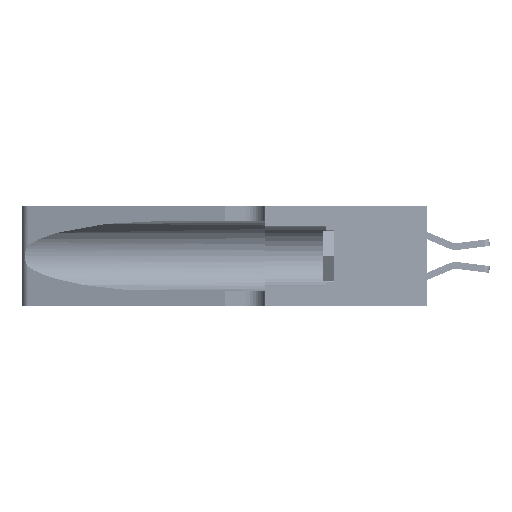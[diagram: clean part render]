
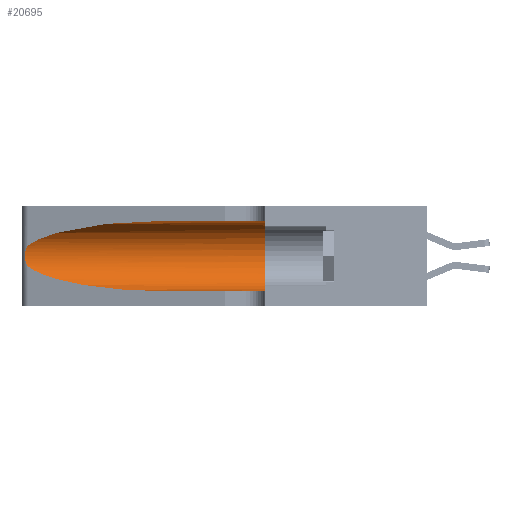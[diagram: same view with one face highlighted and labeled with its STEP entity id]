
A CAD part, left-side view. The second image highlights one B-rep face of the part: STEP entity #20695.
In plain terms, the highlighted cylindrical face has radius 3.308 mm (diameter 6.617 mm), a partial arc.
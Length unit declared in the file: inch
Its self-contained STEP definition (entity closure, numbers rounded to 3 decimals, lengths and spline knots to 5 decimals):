
#72 =( BOUNDED_CURVE ( )  B_SPLINE_CURVE ( 3, ( #38834, #30930, #3303, #15257 ),
 .UNSPECIFIED., .F., .T. ) 
 B_SPLINE_CURVE_WITH_KNOTS ( ( 4, 4 ),
 ( 3.44316, 4.71239 ),
 .UNSPECIFIED. ) 
 CURVE ( )  GEOMETRIC_REPRESENTATION_ITEM ( )  RATIONAL_B_SPLINE_CURVE ( ( 1., 0.87, 0.87, 1. ) ) 
 REPRESENTATION_ITEM ( '' )  );
#582 = CARTESIAN_POINT ( 'NONE',  ( 0.25487, 1.22718, 0.22369 ) ) ;
#637 = VERTEX_POINT ( 'NONE', #31780 ) ;
#1636 = VERTEX_POINT ( 'NONE', #5825 ) ;
#1712 = B_SPLINE_CURVE_WITH_KNOTS ( 'NONE', 3,
 ( #29789, #17929, #37690, #14088, #41618, #18099, #45593, #22097, #49508, #26073, #2306, #29949, #6310, #33889 ),
 .UNSPECIFIED., .F., .F.,
 ( 4, 2, 2, 2, 2, 2, 4 ),
 ( 0., 0.00027, 0.00053, 0.00107, 0.0016, 0.00187, 0.00214 ),
 .UNSPECIFIED. ) ;
#1868 = ORIENTED_EDGE ( 'NONE', *, *, #41012, .T. ) ;
#2306 = CARTESIAN_POINT ( 'NONE',  ( 0.25789, 1.23486, 0.15765 ) ) ;
#2549 = CARTESIAN_POINT ( 'NONE',  ( 0.1305, 0.35, 0.185 ) ) ;
#3303 = CARTESIAN_POINT ( 'NONE',  ( 0.18966, 0.96281, 0.05475 ) ) ;
#3572 = CARTESIAN_POINT ( 'NONE',  ( 0.25487, 1.22718, 0.14631 ) ) ;
#4910 = VECTOR ( 'NONE', #15289, 39.37008 ) ;
#4964 = EDGE_CURVE ( 'NONE', #38314, #37856, #72, .T. ) ;
#5825 = CARTESIAN_POINT ( 'NONE',  ( 0.1305, 0.72297, 0.31525 ) ) ;
#6018 = ORIENTED_EDGE ( 'NONE', *, *, #34022, .T. ) ;
#6310 = CARTESIAN_POINT ( 'NONE',  ( 0.25555, 1.22993, 0.14849 ) ) ;
#6532 = EDGE_LOOP ( 'NONE', ( #1868, #13918, #30629, #6018, #17808, #25780 ) ) ;
#6535 = DIRECTION ( 'NONE',  ( 0., 0., 1. ) ) ;
#7098 = CARTESIAN_POINT ( 'NONE',  ( 0.1305, 1.61858, 0.185 ) ) ;
#7361 = AXIS2_PLACEMENT_3D ( 'NONE', #2549, #30192, #6535 ) ;
#10018 = EDGE_CURVE ( 'NONE', #1636, #637, #36381, .T. ) ;
#10527 = FACE_OUTER_BOUND ( 'NONE', #6532, .T. ) ;
#12421 = CARTESIAN_POINT ( 'NONE',  ( 0.1305, 0.72297, 0.31525 ) ) ;
#12972 = CARTESIAN_POINT ( 'NONE',  ( 0.1305, 0.72297, 0.05475 ) ) ;
#13918 = ORIENTED_EDGE ( 'NONE', *, *, #26414, .T. ) ;
#14088 = CARTESIAN_POINT ( 'NONE',  ( 0.25787, 1.23484, 0.2124 ) ) ;
#15257 = CARTESIAN_POINT ( 'NONE',  ( 0.1305, 0.72297, 0.05475 ) ) ;
#15289 = DIRECTION ( 'NONE',  ( 0., -1., 0. ) ) ;
#16343 =( BOUNDED_CURVE ( )  B_SPLINE_CURVE ( 3, ( #12421, #36013, #24368, #582 ),
 .UNSPECIFIED., .F., .T. ) 
 B_SPLINE_CURVE_WITH_KNOTS ( ( 4, 4 ),
 ( 1.5708, 2.84003 ),
 .UNSPECIFIED. ) 
 CURVE ( )  GEOMETRIC_REPRESENTATION_ITEM ( )  RATIONAL_B_SPLINE_CURVE ( ( 1., 0.87, 0.87, 1. ) ) 
 REPRESENTATION_ITEM ( '' )  );
#17808 = ORIENTED_EDGE ( 'NONE', *, *, #38100, .F. ) ;
#17929 = CARTESIAN_POINT ( 'NONE',  ( 0.25555, 1.22994, 0.2215 ) ) ;
#18099 = CARTESIAN_POINT ( 'NONE',  ( 0.26018, 1.23835, 0.19895 ) ) ;
#20695 = ADVANCED_FACE ( 'NONE', ( #10527 ), #38252, .F. ) ;
#22097 = CARTESIAN_POINT ( 'NONE',  ( 0.26075, 1.23896, 0.178 ) ) ;
#23934 = DIRECTION ( 'NONE',  ( 0., -1., 0. ) ) ;
#24368 = CARTESIAN_POINT ( 'NONE',  ( 0.2373, 1.15595, 0.28018 ) ) ;
#25780 = ORIENTED_EDGE ( 'NONE', *, *, #10018, .F. ) ;
#26073 = CARTESIAN_POINT ( 'NONE',  ( 0.25856, 1.23593, 0.16098 ) ) ;
#26414 = EDGE_CURVE ( 'NONE', #46879, #38314, #1712, .T. ) ;
#27236 = LINE ( 'NONE', #35767, #37652 ) ;
#29789 = CARTESIAN_POINT ( 'NONE',  ( 0.25487, 1.22718, 0.22369 ) ) ;
#29949 = CARTESIAN_POINT ( 'NONE',  ( 0.25639, 1.23186, 0.15144 ) ) ;
#30192 = DIRECTION ( 'NONE',  ( 0., 1., 0. ) ) ;
#30629 = ORIENTED_EDGE ( 'NONE', *, *, #4964, .T. ) ;
#30930 = CARTESIAN_POINT ( 'NONE',  ( 0.2373, 1.15595, 0.08982 ) ) ;
#31780 = CARTESIAN_POINT ( 'NONE',  ( 0.1305, 0.35, 0.31525 ) ) ;
#33508 = CARTESIAN_POINT ( 'NONE',  ( 0.25487, 1.22718, 0.22369 ) ) ;
#33889 = CARTESIAN_POINT ( 'NONE',  ( 0.25487, 1.22718, 0.14631 ) ) ;
#34022 = EDGE_CURVE ( 'NONE', #37856, #47213, #27236, .T. ) ;
#34691 = DIRECTION ( 'NONE',  ( 0., -1., 0. ) ) ;
#35767 = CARTESIAN_POINT ( 'NONE',  ( 0.1305, 1.61858, 0.05475 ) ) ;
#36013 = CARTESIAN_POINT ( 'NONE',  ( 0.18966, 0.96281, 0.31525 ) ) ;
#36381 = LINE ( 'NONE', #42801, #4910 ) ;
#37652 = VECTOR ( 'NONE', #23934, 39.37008 ) ;
#37690 = CARTESIAN_POINT ( 'NONE',  ( 0.25639, 1.23184, 0.21858 ) ) ;
#37856 = VERTEX_POINT ( 'NONE', #12972 ) ;
#38100 = EDGE_CURVE ( 'NONE', #637, #47213, #41975, .T. ) ;
#38252 = CYLINDRICAL_SURFACE ( 'NONE', #39826, 0.13025 ) ;
#38314 = VERTEX_POINT ( 'NONE', #3572 ) ;
#38834 = CARTESIAN_POINT ( 'NONE',  ( 0.25487, 1.22718, 0.14631 ) ) ;
#39826 = AXIS2_PLACEMENT_3D ( 'NONE', #7098, #34691, #42588 ) ;
#41012 = EDGE_CURVE ( 'NONE', #1636, #46879, #16343, .T. ) ;
#41618 = CARTESIAN_POINT ( 'NONE',  ( 0.25854, 1.2359, 0.20912 ) ) ;
#41975 = CIRCLE ( 'NONE', #7361, 0.13025 ) ;
#42588 = DIRECTION ( 'NONE',  ( 0., 0., -1. ) ) ;
#42801 = CARTESIAN_POINT ( 'NONE',  ( 0.1305, 1.61858, 0.31525 ) ) ;
#45593 = CARTESIAN_POINT ( 'NONE',  ( 0.26075, 1.23896, 0.19203 ) ) ;
#46879 = VERTEX_POINT ( 'NONE', #33508 ) ;
#46901 = CARTESIAN_POINT ( 'NONE',  ( 0.1305, 0.35, 0.05475 ) ) ;
#47213 = VERTEX_POINT ( 'NONE', #46901 ) ;
#49508 = CARTESIAN_POINT ( 'NONE',  ( 0.26017, 1.23833, 0.17102 ) ) ;
